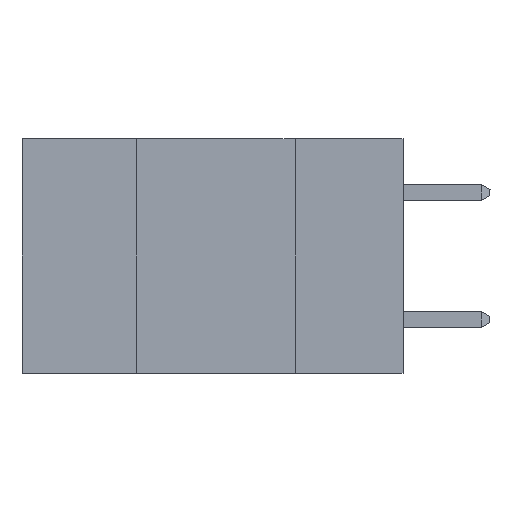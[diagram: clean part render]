
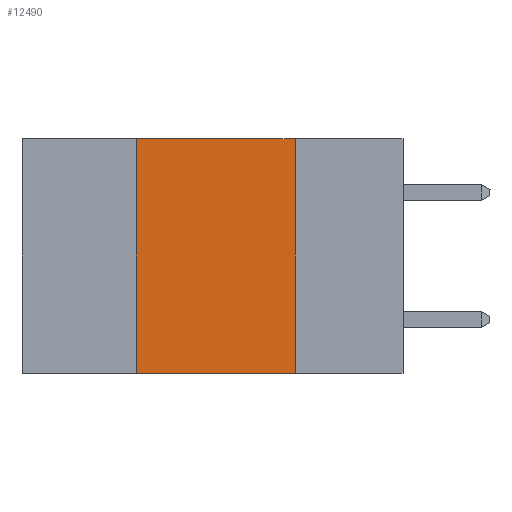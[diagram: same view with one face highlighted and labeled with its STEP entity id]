
A CAD part, left-side view. The second image highlights one B-rep face of the part: STEP entity #12490.
In plain terms, the highlighted planar face has unit normal (-1, 0, 0).
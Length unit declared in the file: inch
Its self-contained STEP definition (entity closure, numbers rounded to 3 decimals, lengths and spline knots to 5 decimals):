
#1410 = EDGE_CURVE ( 'NONE', #4827, #25019, #2326, .T. ) ;
#2213 = EDGE_CURVE ( 'NONE', #4827, #5946, #15370, .T. ) ;
#2326 = LINE ( 'NONE', #10473, #16395 ) ;
#3487 = DIRECTION ( 'NONE',  ( 0., 0., 1. ) ) ;
#3506 = LINE ( 'NONE', #11643, #19747 ) ;
#3564 = AXIS2_PLACEMENT_3D ( 'NONE', #25838, #9685, #24207 ) ;
#3958 = DIRECTION ( 'NONE',  ( 0., 0., -1. ) ) ;
#4827 = VERTEX_POINT ( 'NONE', #13141 ) ;
#5946 = VERTEX_POINT ( 'NONE', #18557 ) ;
#6707 = EDGE_LOOP ( 'NONE', ( #24852, #7540, #10938, #7573 ) ) ;
#7540 = ORIENTED_EDGE ( 'NONE', *, *, #11068, .F. ) ;
#7573 = ORIENTED_EDGE ( 'NONE', *, *, #1410, .T. ) ;
#8304 = EDGE_CURVE ( 'NONE', #20283, #25019, #18111, .T. ) ;
#9259 = DIRECTION ( 'NONE',  ( 0., -1., 0. ) ) ;
#9631 = CARTESIAN_POINT ( 'NONE',  ( 0., 0.17, 0. ) ) ;
#9685 = DIRECTION ( 'NONE',  ( 1., 0., 0. ) ) ;
#10473 = CARTESIAN_POINT ( 'NONE',  ( 0., 0.6, -0.37 ) ) ;
#10938 = ORIENTED_EDGE ( 'NONE', *, *, #2213, .F. ) ;
#11068 = EDGE_CURVE ( 'NONE', #5946, #20283, #3506, .T. ) ;
#11643 = CARTESIAN_POINT ( 'NONE',  ( 0., 0.6, 0. ) ) ;
#12490 = ADVANCED_FACE ( 'NONE', ( #17689 ), #15825, .F. ) ;
#13141 = CARTESIAN_POINT ( 'NONE',  ( 0., 0.42, -0.37 ) ) ;
#15002 = CARTESIAN_POINT ( 'NONE',  ( 0., 0.17, -0.37 ) ) ;
#15370 = LINE ( 'NONE', #25510, #23185 ) ;
#15825 = PLANE ( 'NONE',  #3564 ) ;
#15842 = VECTOR ( 'NONE', #3958, 39.37008 ) ;
#16395 = VECTOR ( 'NONE', #20478, 39.37008 ) ;
#17689 = FACE_OUTER_BOUND ( 'NONE', #6707, .T. ) ;
#18111 = LINE ( 'NONE', #26259, #15842 ) ;
#18557 = CARTESIAN_POINT ( 'NONE',  ( 0., 0.42, 0. ) ) ;
#19747 = VECTOR ( 'NONE', #9259, 39.37008 ) ;
#20283 = VERTEX_POINT ( 'NONE', #9631 ) ;
#20478 = DIRECTION ( 'NONE',  ( 0., -1., 0. ) ) ;
#23185 = VECTOR ( 'NONE', #3487, 39.37008 ) ;
#24207 = DIRECTION ( 'NONE',  ( 0., 0., -1. ) ) ;
#24852 = ORIENTED_EDGE ( 'NONE', *, *, #8304, .F. ) ;
#25019 = VERTEX_POINT ( 'NONE', #15002 ) ;
#25510 = CARTESIAN_POINT ( 'NONE',  ( 0., 0.42, 0. ) ) ;
#25838 = CARTESIAN_POINT ( 'NONE',  ( 0., 0.6, 0. ) ) ;
#26259 = CARTESIAN_POINT ( 'NONE',  ( 0., 0.17, 0. ) ) ;
